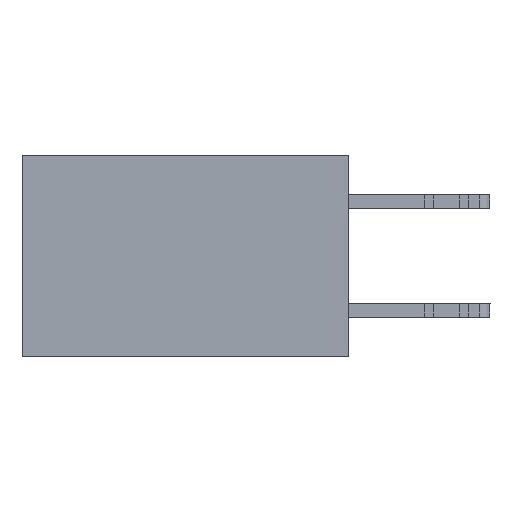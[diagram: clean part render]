
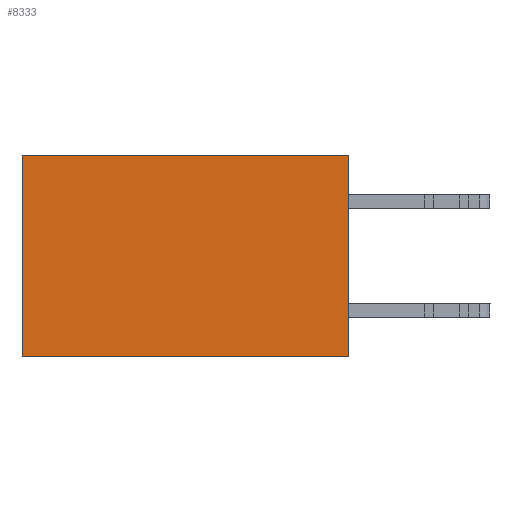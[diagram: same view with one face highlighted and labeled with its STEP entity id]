
A CAD part, left-side view. The second image highlights one B-rep face of the part: STEP entity #8333.
In plain terms, the highlighted planar face has unit normal (-1, 0, 0).
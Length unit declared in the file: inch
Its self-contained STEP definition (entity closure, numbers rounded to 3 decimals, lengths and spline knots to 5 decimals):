
#28 = VERTEX_POINT ( 'NONE', #20746 ) ;
#61 = DIRECTION ( 'NONE',  ( 1., 0., 0. ) ) ;
#2715 = CARTESIAN_POINT ( 'NONE',  ( 0.2615, 0., -0.37 ) ) ;
#2981 = CARTESIAN_POINT ( 'NONE',  ( 0.2615, 0., 0. ) ) ;
#3298 = VERTEX_POINT ( 'NONE', #2981 ) ;
#4251 = ORIENTED_EDGE ( 'NONE', *, *, #24131, .T. ) ;
#7770 = DIRECTION ( 'NONE',  ( 0., 1., 0. ) ) ;
#8333 = ADVANCED_FACE ( 'NONE', ( #15203 ), #10684, .F. ) ;
#9354 = EDGE_CURVE ( 'NONE', #13914, #28, #10346, .T. ) ;
#9534 = ORIENTED_EDGE ( 'NONE', *, *, #12774, .F. ) ;
#9933 = CARTESIAN_POINT ( 'NONE',  ( 0.2615, 0., 0. ) ) ;
#10083 = DIRECTION ( 'NONE',  ( 0., 1., 0. ) ) ;
#10346 = LINE ( 'NONE', #14374, #15345 ) ;
#10586 = CARTESIAN_POINT ( 'NONE',  ( 0.2615, 0.6, -0.37 ) ) ;
#10684 = PLANE ( 'NONE',  #18894 ) ;
#11561 = LINE ( 'NONE', #2715, #22758 ) ;
#12448 = VECTOR ( 'NONE', #7770, 39.37008 ) ;
#12774 = EDGE_CURVE ( 'NONE', #3298, #13914, #11561, .T. ) ;
#12814 = VERTEX_POINT ( 'NONE', #15551 ) ;
#12921 = CARTESIAN_POINT ( 'NONE',  ( 0.2615, 0., -0.37 ) ) ;
#13144 = LINE ( 'NONE', #9933, #12448 ) ;
#13157 = LINE ( 'NONE', #10586, #24274 ) ;
#13914 = VERTEX_POINT ( 'NONE', #12921 ) ;
#14374 = CARTESIAN_POINT ( 'NONE',  ( 0.2615, 0., -0.37 ) ) ;
#14968 = DIRECTION ( 'NONE',  ( 0., 0., -1. ) ) ;
#15203 = FACE_OUTER_BOUND ( 'NONE', #22560, .T. ) ;
#15345 = VECTOR ( 'NONE', #10083, 39.37008 ) ;
#15455 = DIRECTION ( 'NONE',  ( 0., 0., -1. ) ) ;
#15551 = CARTESIAN_POINT ( 'NONE',  ( 0.2615, 0.6, 0. ) ) ;
#17701 = EDGE_CURVE ( 'NONE', #3298, #12814, #13144, .T. ) ;
#18894 = AXIS2_PLACEMENT_3D ( 'NONE', #25334, #61, #14968 ) ;
#19677 = ORIENTED_EDGE ( 'NONE', *, *, #9354, .F. ) ;
#20746 = CARTESIAN_POINT ( 'NONE',  ( 0.2615, 0.6, -0.37 ) ) ;
#22560 = EDGE_LOOP ( 'NONE', ( #4251, #19677, #9534, #23395 ) ) ;
#22758 = VECTOR ( 'NONE', #15455, 39.37008 ) ;
#23395 = ORIENTED_EDGE ( 'NONE', *, *, #17701, .T. ) ;
#24131 = EDGE_CURVE ( 'NONE', #12814, #28, #13157, .T. ) ;
#24274 = VECTOR ( 'NONE', #25241, 39.37008 ) ;
#25241 = DIRECTION ( 'NONE',  ( 0., 0., -1. ) ) ;
#25334 = CARTESIAN_POINT ( 'NONE',  ( 0.2615, 0., -0.37 ) ) ;
